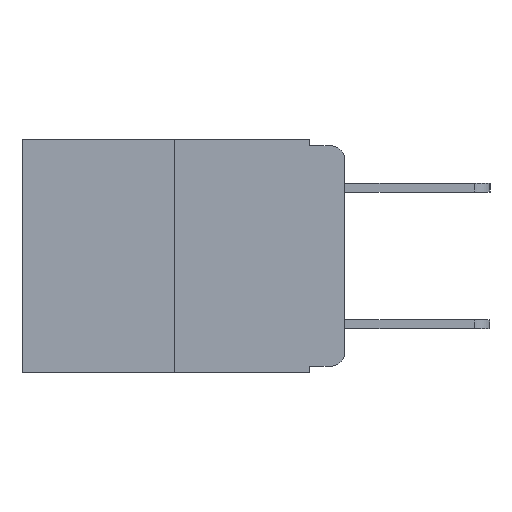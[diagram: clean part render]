
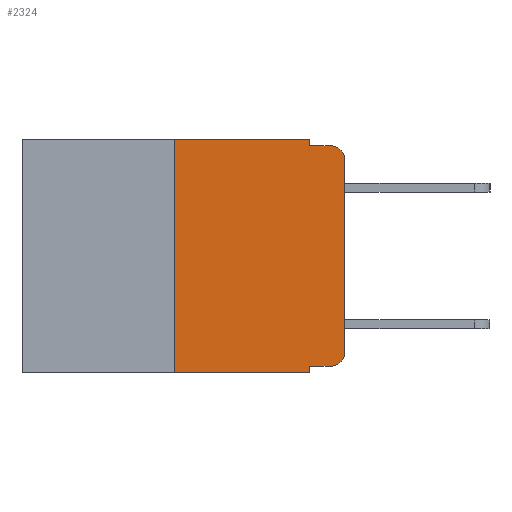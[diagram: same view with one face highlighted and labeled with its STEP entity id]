
A CAD part, left-side view. The second image highlights one B-rep face of the part: STEP entity #2324.
In plain terms, the highlighted planar face has unit normal (-1, 0, 0).
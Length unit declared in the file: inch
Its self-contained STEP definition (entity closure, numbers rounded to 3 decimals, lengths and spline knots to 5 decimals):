
#167 = EDGE_CURVE ( 'NONE', #431, #4180, #9335, .T. ) ;
#174 = VERTEX_POINT ( 'NONE', #6297 ) ;
#431 = VERTEX_POINT ( 'NONE', #5392 ) ;
#571 = LINE ( 'NONE', #3532, #899 ) ;
#581 = LINE ( 'NONE', #6573, #9919 ) ;
#899 = VECTOR ( 'NONE', #3127, 39.37008 ) ;
#1232 = LINE ( 'NONE', #7362, #8796 ) ;
#1404 = VERTEX_POINT ( 'NONE', #4279 ) ;
#1677 = AXIS2_PLACEMENT_3D ( 'NONE', #8531, #4061, #6009 ) ;
#1809 = EDGE_LOOP ( 'NONE', ( #11462, #9863, #11088, #10002, #3344, #8627, #7442, #9873, #5620, #4354 ) ) ;
#2073 = EDGE_CURVE ( 'NONE', #9833, #7311, #10058, .T. ) ;
#2132 = CARTESIAN_POINT ( 'NONE',  ( 0., 0.473, 0. ) ) ;
#2200 = EDGE_CURVE ( 'NONE', #174, #8492, #1232, .T. ) ;
#2236 = EDGE_CURVE ( 'NONE', #6048, #10034, #581, .T. ) ;
#2241 = VECTOR ( 'NONE', #5570, 39.37008 ) ;
#2252 = EDGE_CURVE ( 'NONE', #10034, #5805, #5396, .T. ) ;
#2324 = ADVANCED_FACE ( 'NONE', ( #4264 ), #7713, .F. ) ;
#2554 = EDGE_CURVE ( 'NONE', #9833, #431, #8550, .T. ) ;
#2575 = EDGE_CURVE ( 'NONE', #6048, #7311, #571, .T. ) ;
#2675 = DIRECTION ( 'NONE',  ( 0., 0., 1. ) ) ;
#2891 = DIRECTION ( 'NONE',  ( 0., 0., -1. ) ) ;
#2903 = DIRECTION ( 'NONE',  ( -1., 0., 0. ) ) ;
#3045 = EDGE_CURVE ( 'NONE', #1404, #8492, #4244, .T. ) ;
#3127 = DIRECTION ( 'NONE',  ( 0., 0., -1. ) ) ;
#3256 = VECTOR ( 'NONE', #2891, 39.37008 ) ;
#3344 = ORIENTED_EDGE ( 'NONE', *, *, #167, .F. ) ;
#3532 = CARTESIAN_POINT ( 'NONE',  ( 0., 0.051, 0. ) ) ;
#3538 = VECTOR ( 'NONE', #2675, 39.37008 ) ;
#3846 = LINE ( 'NONE', #9076, #3256 ) ;
#4001 = DIRECTION ( 'NONE',  ( 0., -1., 0. ) ) ;
#4061 = DIRECTION ( 'NONE',  ( -1., 0., 0. ) ) ;
#4180 = VERTEX_POINT ( 'NONE', #11405 ) ;
#4244 = CIRCLE ( 'NONE', #7366, 0.02 ) ;
#4264 = FACE_OUTER_BOUND ( 'NONE', #1809, .T. ) ;
#4279 = CARTESIAN_POINT ( 'NONE',  ( 0., 0., -0.03 ) ) ;
#4354 = ORIENTED_EDGE ( 'NONE', *, *, #2252, .T. ) ;
#4970 = EDGE_CURVE ( 'NONE', #5805, #1404, #6245, .T. ) ;
#4985 = DIRECTION ( 'NONE',  ( 0., -1., 0. ) ) ;
#5392 = CARTESIAN_POINT ( 'NONE',  ( 0., 0.25, 0. ) ) ;
#5396 = CIRCLE ( 'NONE', #1677, 0.02 ) ;
#5468 = EDGE_CURVE ( 'NONE', #4180, #174, #3846, .T. ) ;
#5536 = VECTOR ( 'NONE', #4985, 39.37008 ) ;
#5570 = DIRECTION ( 'NONE',  ( 0., -1., 0. ) ) ;
#5620 = ORIENTED_EDGE ( 'NONE', *, *, #2236, .T. ) ;
#5717 = CARTESIAN_POINT ( 'NONE',  ( 0., 0.051, -0.333 ) ) ;
#5732 = CARTESIAN_POINT ( 'NONE',  ( 0., 0., 0. ) ) ;
#5805 = VERTEX_POINT ( 'NONE', #9599 ) ;
#6009 = DIRECTION ( 'NONE',  ( 0., 0., -1. ) ) ;
#6048 = VERTEX_POINT ( 'NONE', #5717 ) ;
#6105 = CARTESIAN_POINT ( 'NONE',  ( 0., 0.25, -0.343 ) ) ;
#6245 = LINE ( 'NONE', #5732, #8567 ) ;
#6288 = CARTESIAN_POINT ( 'NONE',  ( 0., 0.02, -0.333 ) ) ;
#6297 = CARTESIAN_POINT ( 'NONE',  ( 0., 0.051, -0.01 ) ) ;
#6573 = CARTESIAN_POINT ( 'NONE',  ( 0., 0.051, -0.333 ) ) ;
#6675 = DIRECTION ( 'NONE',  ( 0., 0., 1. ) ) ;
#7287 = AXIS2_PLACEMENT_3D ( 'NONE', #2132, #7686, #8939 ) ;
#7311 = VERTEX_POINT ( 'NONE', #11325 ) ;
#7362 = CARTESIAN_POINT ( 'NONE',  ( 0., 0.051, -0.01 ) ) ;
#7366 = AXIS2_PLACEMENT_3D ( 'NONE', #8284, #2903, #9088 ) ;
#7442 = ORIENTED_EDGE ( 'NONE', *, *, #2073, .T. ) ;
#7686 = DIRECTION ( 'NONE',  ( 1., 0., 0. ) ) ;
#7713 = PLANE ( 'NONE',  #7287 ) ;
#8284 = CARTESIAN_POINT ( 'NONE',  ( 0., 0.02, -0.03 ) ) ;
#8492 = VERTEX_POINT ( 'NONE', #8711 ) ;
#8531 = CARTESIAN_POINT ( 'NONE',  ( 0., 0.02, -0.313 ) ) ;
#8550 = LINE ( 'NONE', #9255, #3538 ) ;
#8567 = VECTOR ( 'NONE', #6675, 39.37008 ) ;
#8627 = ORIENTED_EDGE ( 'NONE', *, *, #2554, .F. ) ;
#8711 = CARTESIAN_POINT ( 'NONE',  ( 0., 0.02, -0.01 ) ) ;
#8796 = VECTOR ( 'NONE', #9230, 39.37008 ) ;
#8939 = DIRECTION ( 'NONE',  ( 0., 0., -1. ) ) ;
#9076 = CARTESIAN_POINT ( 'NONE',  ( 0., 0.051, 0. ) ) ;
#9088 = DIRECTION ( 'NONE',  ( 0., 0., -1. ) ) ;
#9230 = DIRECTION ( 'NONE',  ( 0., -1., 0. ) ) ;
#9255 = CARTESIAN_POINT ( 'NONE',  ( 0., 0.25, 0. ) ) ;
#9335 = LINE ( 'NONE', #10479, #2241 ) ;
#9599 = CARTESIAN_POINT ( 'NONE',  ( 0., 0., -0.313 ) ) ;
#9655 = CARTESIAN_POINT ( 'NONE',  ( 0., 0.473, -0.343 ) ) ;
#9833 = VERTEX_POINT ( 'NONE', #6105 ) ;
#9863 = ORIENTED_EDGE ( 'NONE', *, *, #3045, .T. ) ;
#9873 = ORIENTED_EDGE ( 'NONE', *, *, #2575, .F. ) ;
#9919 = VECTOR ( 'NONE', #4001, 39.37008 ) ;
#10002 = ORIENTED_EDGE ( 'NONE', *, *, #5468, .F. ) ;
#10034 = VERTEX_POINT ( 'NONE', #6288 ) ;
#10058 = LINE ( 'NONE', #9655, #5536 ) ;
#10479 = CARTESIAN_POINT ( 'NONE',  ( 0., 0.473, 0. ) ) ;
#11088 = ORIENTED_EDGE ( 'NONE', *, *, #2200, .F. ) ;
#11325 = CARTESIAN_POINT ( 'NONE',  ( 0., 0.051, -0.343 ) ) ;
#11405 = CARTESIAN_POINT ( 'NONE',  ( 0., 0.051, 0. ) ) ;
#11462 = ORIENTED_EDGE ( 'NONE', *, *, #4970, .T. ) ;
